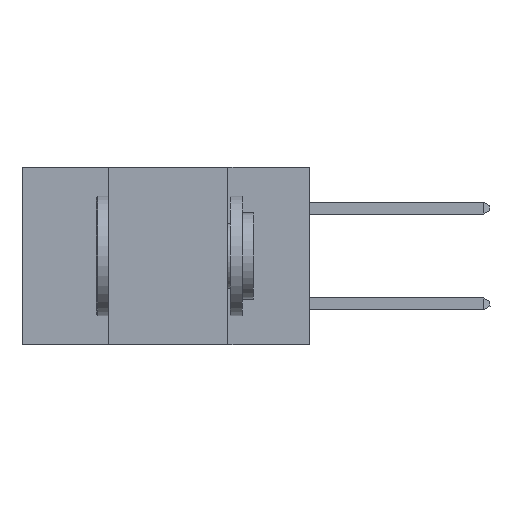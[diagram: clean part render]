
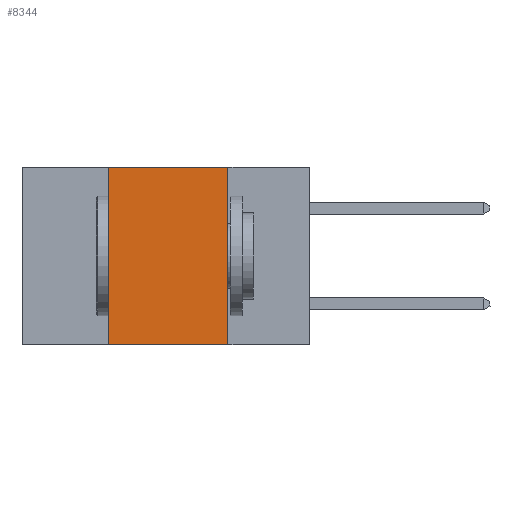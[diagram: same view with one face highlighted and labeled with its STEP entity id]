
A CAD part, left-side view. The second image highlights one B-rep face of the part: STEP entity #8344.
In plain terms, the highlighted planar face has unit normal (-1, 0, 0).
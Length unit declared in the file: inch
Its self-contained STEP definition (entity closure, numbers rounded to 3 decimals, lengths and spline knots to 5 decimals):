
#252 = CARTESIAN_POINT ( 'NONE',  ( 0., 0.17, 0. ) ) ;
#383 = DIRECTION ( 'NONE',  ( 0., 0., 1. ) ) ;
#448 = EDGE_CURVE ( 'NONE', #729, #10879, #7855, .T. ) ;
#729 = VERTEX_POINT ( 'NONE', #12651 ) ;
#891 = DIRECTION ( 'NONE',  ( 0., -1., 0. ) ) ;
#952 = DIRECTION ( 'NONE',  ( 1., 0., 0. ) ) ;
#1078 = VERTEX_POINT ( 'NONE', #6265 ) ;
#1280 = CARTESIAN_POINT ( 'NONE',  ( 0., 0.6, -0.37 ) ) ;
#1861 = EDGE_CURVE ( 'NONE', #729, #2763, #7087, .T. ) ;
#2374 = DIRECTION ( 'NONE',  ( 0., 0., -1. ) ) ;
#2763 = VERTEX_POINT ( 'NONE', #6472 ) ;
#2982 = CARTESIAN_POINT ( 'NONE',  ( 0., 0.6, 0. ) ) ;
#3963 = LINE ( 'NONE', #252, #6307 ) ;
#4135 = DIRECTION ( 'NONE',  ( 0., -1., 0. ) ) ;
#4408 = VECTOR ( 'NONE', #383, 39.37008 ) ;
#6265 = CARTESIAN_POINT ( 'NONE',  ( 0., 0.17, 0. ) ) ;
#6307 = VECTOR ( 'NONE', #2374, 39.37008 ) ;
#6431 = EDGE_LOOP ( 'NONE', ( #6771, #7097, #12445, #7904 ) ) ;
#6472 = CARTESIAN_POINT ( 'NONE',  ( 0., 0.42, 0. ) ) ;
#6509 = CARTESIAN_POINT ( 'NONE',  ( 0., 0.17, -0.37 ) ) ;
#6550 = LINE ( 'NONE', #11060, #12100 ) ;
#6771 = ORIENTED_EDGE ( 'NONE', *, *, #7955, .F. ) ;
#7002 = PLANE ( 'NONE',  #8506 ) ;
#7087 = LINE ( 'NONE', #12149, #4408 ) ;
#7097 = ORIENTED_EDGE ( 'NONE', *, *, #11262, .F. ) ;
#7564 = FACE_OUTER_BOUND ( 'NONE', #6431, .T. ) ;
#7855 = LINE ( 'NONE', #1280, #12731 ) ;
#7904 = ORIENTED_EDGE ( 'NONE', *, *, #448, .T. ) ;
#7955 = EDGE_CURVE ( 'NONE', #1078, #10879, #3963, .T. ) ;
#8033 = DIRECTION ( 'NONE',  ( 0., 0., -1. ) ) ;
#8344 = ADVANCED_FACE ( 'NONE', ( #7564 ), #7002, .F. ) ;
#8506 = AXIS2_PLACEMENT_3D ( 'NONE', #2982, #952, #8033 ) ;
#10879 = VERTEX_POINT ( 'NONE', #6509 ) ;
#11060 = CARTESIAN_POINT ( 'NONE',  ( 0., 0.6, 0. ) ) ;
#11262 = EDGE_CURVE ( 'NONE', #2763, #1078, #6550, .T. ) ;
#12100 = VECTOR ( 'NONE', #4135, 39.37008 ) ;
#12149 = CARTESIAN_POINT ( 'NONE',  ( 0., 0.42, 0. ) ) ;
#12445 = ORIENTED_EDGE ( 'NONE', *, *, #1861, .F. ) ;
#12651 = CARTESIAN_POINT ( 'NONE',  ( 0., 0.42, -0.37 ) ) ;
#12731 = VECTOR ( 'NONE', #891, 39.37008 ) ;
